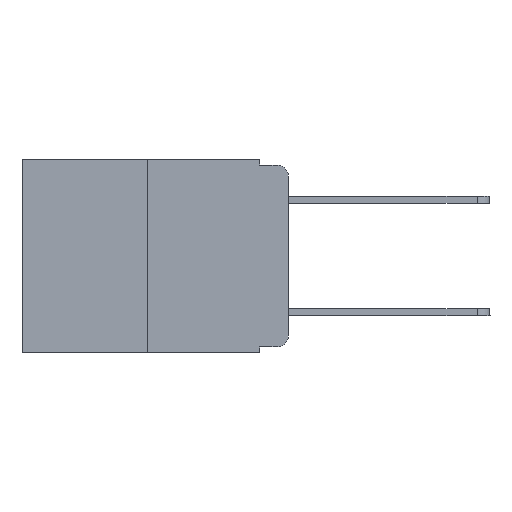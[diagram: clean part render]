
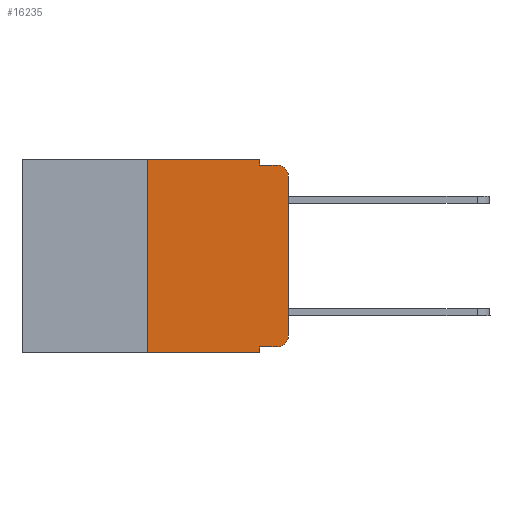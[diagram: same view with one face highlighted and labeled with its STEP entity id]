
A CAD part, left-side view. The second image highlights one B-rep face of the part: STEP entity #16235.
In plain terms, the highlighted planar face has unit normal (-1, 0, 0).
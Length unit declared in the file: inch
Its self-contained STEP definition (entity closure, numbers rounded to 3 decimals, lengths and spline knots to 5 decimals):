
#313 = CARTESIAN_POINT ( 'NONE',  ( 0., 0.473, 0. ) ) ;
#370 = CARTESIAN_POINT ( 'NONE',  ( 0., 0.02, -0.313 ) ) ;
#653 = VERTEX_POINT ( 'NONE', #6774 ) ;
#702 = CARTESIAN_POINT ( 'NONE',  ( 0., 0.02, -0.01 ) ) ;
#844 = EDGE_CURVE ( 'NONE', #9610, #11777, #6854, .T. ) ;
#1139 = DIRECTION ( 'NONE',  ( 0., -1., 0. ) ) ;
#1186 = CARTESIAN_POINT ( 'NONE',  ( 0., 0.051, -0.333 ) ) ;
#1353 = AXIS2_PLACEMENT_3D ( 'NONE', #13448, #15108, #6591 ) ;
#1578 = LINE ( 'NONE', #3358, #3119 ) ;
#1954 = EDGE_CURVE ( 'NONE', #12683, #653, #16727, .T. ) ;
#2033 = ORIENTED_EDGE ( 'NONE', *, *, #17540, .T. ) ;
#2169 = CARTESIAN_POINT ( 'NONE',  ( 0., 0.051, -0.01 ) ) ;
#3118 = DIRECTION ( 'NONE',  ( 0., 0., -1. ) ) ;
#3119 = VECTOR ( 'NONE', #4575, 39.37008 ) ;
#3339 = DIRECTION ( 'NONE',  ( 1., 0., 0. ) ) ;
#3358 = CARTESIAN_POINT ( 'NONE',  ( 0., 0.051, 0. ) ) ;
#3386 = EDGE_CURVE ( 'NONE', #7058, #8293, #7991, .T. ) ;
#3686 = LINE ( 'NONE', #9463, #7575 ) ;
#4013 = LINE ( 'NONE', #8856, #4237 ) ;
#4237 = VECTOR ( 'NONE', #16146, 39.37008 ) ;
#4575 = DIRECTION ( 'NONE',  ( 0., 0., -1. ) ) ;
#4657 = EDGE_CURVE ( 'NONE', #8293, #6770, #14983, .T. ) ;
#4820 = ORIENTED_EDGE ( 'NONE', *, *, #844, .F. ) ;
#5455 = ORIENTED_EDGE ( 'NONE', *, *, #8759, .T. ) ;
#5794 = EDGE_CURVE ( 'NONE', #11777, #7058, #4013, .T. ) ;
#6109 = VERTEX_POINT ( 'NONE', #9232 ) ;
#6482 = EDGE_CURVE ( 'NONE', #6109, #12683, #12732, .T. ) ;
#6591 = DIRECTION ( 'NONE',  ( 0., 0., -1. ) ) ;
#6770 = VERTEX_POINT ( 'NONE', #702 ) ;
#6774 = CARTESIAN_POINT ( 'NONE',  ( 0., 0., -0.03 ) ) ;
#6854 = LINE ( 'NONE', #11091, #12325 ) ;
#6898 = ORIENTED_EDGE ( 'NONE', *, *, #3386, .F. ) ;
#7058 = VERTEX_POINT ( 'NONE', #17991 ) ;
#7432 = VERTEX_POINT ( 'NONE', #8214 ) ;
#7575 = VECTOR ( 'NONE', #1139, 39.37008 ) ;
#7991 = LINE ( 'NONE', #16653, #17898 ) ;
#8178 = DIRECTION ( 'NONE',  ( 0., 0., 1. ) ) ;
#8214 = CARTESIAN_POINT ( 'NONE',  ( 0., 0.051, -0.343 ) ) ;
#8293 = VERTEX_POINT ( 'NONE', #2169 ) ;
#8615 = EDGE_CURVE ( 'NONE', #16926, #6109, #3686, .T. ) ;
#8759 = EDGE_CURVE ( 'NONE', #9610, #7432, #14848, .T. ) ;
#8824 = CARTESIAN_POINT ( 'NONE',  ( 0., 0.473, -0.343 ) ) ;
#8856 = CARTESIAN_POINT ( 'NONE',  ( 0., 0.473, 0. ) ) ;
#9232 = CARTESIAN_POINT ( 'NONE',  ( 0., 0.02, -0.333 ) ) ;
#9463 = CARTESIAN_POINT ( 'NONE',  ( 0., 0.051, -0.333 ) ) ;
#9610 = VERTEX_POINT ( 'NONE', #14797 ) ;
#9698 = EDGE_LOOP ( 'NONE', ( #12706, #2033, #12327, #6898, #15971, #4820, #5455, #12828, #15536, #14646 ) ) ;
#9926 = DIRECTION ( 'NONE',  ( 0., 0., -1. ) ) ;
#10005 = PLANE ( 'NONE',  #17510 ) ;
#10191 = CARTESIAN_POINT ( 'NONE',  ( 0., 0.25, 0. ) ) ;
#10416 = VECTOR ( 'NONE', #17246, 39.37008 ) ;
#11091 = CARTESIAN_POINT ( 'NONE',  ( 0., 0.25, 0. ) ) ;
#11237 = CARTESIAN_POINT ( 'NONE',  ( 0., 0., -0.313 ) ) ;
#11622 = CARTESIAN_POINT ( 'NONE',  ( 0., 0.051, -0.01 ) ) ;
#11696 = AXIS2_PLACEMENT_3D ( 'NONE', #370, #17067, #3118 ) ;
#11777 = VERTEX_POINT ( 'NONE', #10191 ) ;
#11967 = FACE_OUTER_BOUND ( 'NONE', #9698, .T. ) ;
#12325 = VECTOR ( 'NONE', #12518, 39.37008 ) ;
#12327 = ORIENTED_EDGE ( 'NONE', *, *, #4657, .F. ) ;
#12518 = DIRECTION ( 'NONE',  ( 0., 0., 1. ) ) ;
#12683 = VERTEX_POINT ( 'NONE', #11237 ) ;
#12706 = ORIENTED_EDGE ( 'NONE', *, *, #1954, .T. ) ;
#12732 = CIRCLE ( 'NONE', #11696, 0.02 ) ;
#12828 = ORIENTED_EDGE ( 'NONE', *, *, #14625, .F. ) ;
#13098 = DIRECTION ( 'NONE',  ( 0., 0., -1. ) ) ;
#13448 = CARTESIAN_POINT ( 'NONE',  ( 0., 0.02, -0.03 ) ) ;
#13589 = CARTESIAN_POINT ( 'NONE',  ( 0., 0., 0. ) ) ;
#13870 = VECTOR ( 'NONE', #8178, 39.37008 ) ;
#14105 = VECTOR ( 'NONE', #17205, 39.37008 ) ;
#14625 = EDGE_CURVE ( 'NONE', #16926, #7432, #1578, .T. ) ;
#14646 = ORIENTED_EDGE ( 'NONE', *, *, #6482, .T. ) ;
#14797 = CARTESIAN_POINT ( 'NONE',  ( 0., 0.25, -0.343 ) ) ;
#14848 = LINE ( 'NONE', #8824, #10416 ) ;
#14983 = LINE ( 'NONE', #11622, #14105 ) ;
#15108 = DIRECTION ( 'NONE',  ( -1., 0., 0. ) ) ;
#15536 = ORIENTED_EDGE ( 'NONE', *, *, #8615, .T. ) ;
#15971 = ORIENTED_EDGE ( 'NONE', *, *, #5794, .F. ) ;
#16146 = DIRECTION ( 'NONE',  ( 0., -1., 0. ) ) ;
#16235 = ADVANCED_FACE ( 'NONE', ( #11967 ), #10005, .F. ) ;
#16653 = CARTESIAN_POINT ( 'NONE',  ( 0., 0.051, 0. ) ) ;
#16727 = LINE ( 'NONE', #13589, #13870 ) ;
#16833 = CIRCLE ( 'NONE', #1353, 0.02 ) ;
#16926 = VERTEX_POINT ( 'NONE', #1186 ) ;
#17067 = DIRECTION ( 'NONE',  ( -1., 0., 0. ) ) ;
#17205 = DIRECTION ( 'NONE',  ( 0., -1., 0. ) ) ;
#17246 = DIRECTION ( 'NONE',  ( 0., -1., 0. ) ) ;
#17510 = AXIS2_PLACEMENT_3D ( 'NONE', #313, #3339, #13098 ) ;
#17540 = EDGE_CURVE ( 'NONE', #653, #6770, #16833, .T. ) ;
#17898 = VECTOR ( 'NONE', #9926, 39.37008 ) ;
#17991 = CARTESIAN_POINT ( 'NONE',  ( 0., 0.051, 0. ) ) ;
